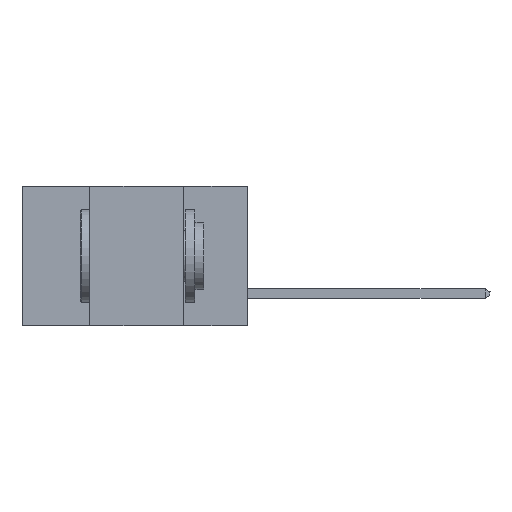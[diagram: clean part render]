
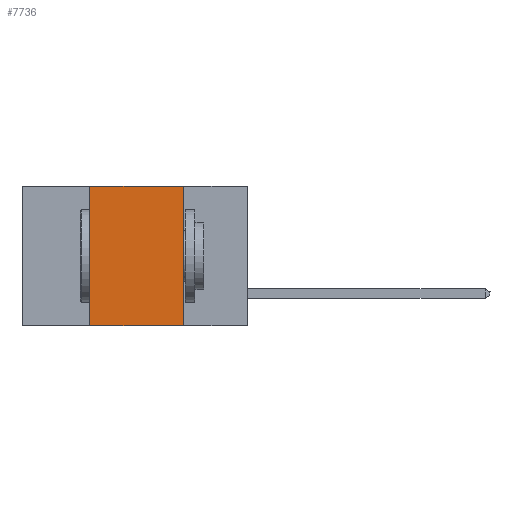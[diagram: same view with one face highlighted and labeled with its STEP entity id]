
A CAD part, left-side view. The second image highlights one B-rep face of the part: STEP entity #7736.
In plain terms, the highlighted planar face has unit normal (-1, 0, 0).
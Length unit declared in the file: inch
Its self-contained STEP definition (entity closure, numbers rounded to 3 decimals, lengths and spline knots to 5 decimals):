
#1212 = EDGE_CURVE ( 'NONE', #19914, #11761, #7031, .T. ) ;
#1830 = CARTESIAN_POINT ( 'NONE',  ( 0., 0.6, 0. ) ) ;
#2474 = EDGE_LOOP ( 'NONE', ( #18633, #15287, #23912, #4804 ) ) ;
#3505 = EDGE_CURVE ( 'NONE', #19317, #11761, #18135, .T. ) ;
#3615 = DIRECTION ( 'NONE',  ( 1., 0., 0. ) ) ;
#3740 = EDGE_CURVE ( 'NONE', #19317, #4763, #24353, .T. ) ;
#4254 = VECTOR ( 'NONE', #20774, 39.37008 ) ;
#4763 = VERTEX_POINT ( 'NONE', #8212 ) ;
#4804 = ORIENTED_EDGE ( 'NONE', *, *, #3505, .T. ) ;
#5337 = DIRECTION ( 'NONE',  ( 0., -1., 0. ) ) ;
#7031 = LINE ( 'NONE', #17004, #4254 ) ;
#7736 = ADVANCED_FACE ( 'NONE', ( #17214 ), #11247, .F. ) ;
#8212 = CARTESIAN_POINT ( 'NONE',  ( 0., 0.42, 0. ) ) ;
#10595 = AXIS2_PLACEMENT_3D ( 'NONE', #1830, #3615, #11507 ) ;
#11247 = PLANE ( 'NONE',  #10595 ) ;
#11507 = DIRECTION ( 'NONE',  ( 0., 0., -1. ) ) ;
#11761 = VERTEX_POINT ( 'NONE', #14031 ) ;
#12212 = CARTESIAN_POINT ( 'NONE',  ( 0., 0.42, -0.37 ) ) ;
#13198 = VECTOR ( 'NONE', #24208, 39.37008 ) ;
#14028 = DIRECTION ( 'NONE',  ( 0., 0., 1. ) ) ;
#14031 = CARTESIAN_POINT ( 'NONE',  ( 0., 0.17, -0.37 ) ) ;
#15287 = ORIENTED_EDGE ( 'NONE', *, *, #24417, .F. ) ;
#16314 = VECTOR ( 'NONE', #5337, 39.37008 ) ;
#16358 = CARTESIAN_POINT ( 'NONE',  ( 0., 0.6, -0.37 ) ) ;
#17004 = CARTESIAN_POINT ( 'NONE',  ( 0., 0.17, -0.37 ) ) ;
#17214 = FACE_OUTER_BOUND ( 'NONE', #2474, .T. ) ;
#18135 = LINE ( 'NONE', #16358, #13198 ) ;
#18633 = ORIENTED_EDGE ( 'NONE', *, *, #1212, .F. ) ;
#19317 = VERTEX_POINT ( 'NONE', #23607 ) ;
#19914 = VERTEX_POINT ( 'NONE', #25348 ) ;
#20774 = DIRECTION ( 'NONE',  ( 0., 0., -1. ) ) ;
#20886 = LINE ( 'NONE', #23064, #16314 ) ;
#21894 = VECTOR ( 'NONE', #14028, 39.37008 ) ;
#23064 = CARTESIAN_POINT ( 'NONE',  ( 0., 0.6, 0. ) ) ;
#23607 = CARTESIAN_POINT ( 'NONE',  ( 0., 0.42, -0.37 ) ) ;
#23912 = ORIENTED_EDGE ( 'NONE', *, *, #3740, .F. ) ;
#24208 = DIRECTION ( 'NONE',  ( 0., -1., 0. ) ) ;
#24353 = LINE ( 'NONE', #12212, #21894 ) ;
#24417 = EDGE_CURVE ( 'NONE', #4763, #19914, #20886, .T. ) ;
#25348 = CARTESIAN_POINT ( 'NONE',  ( 0., 0.17, 0. ) ) ;
